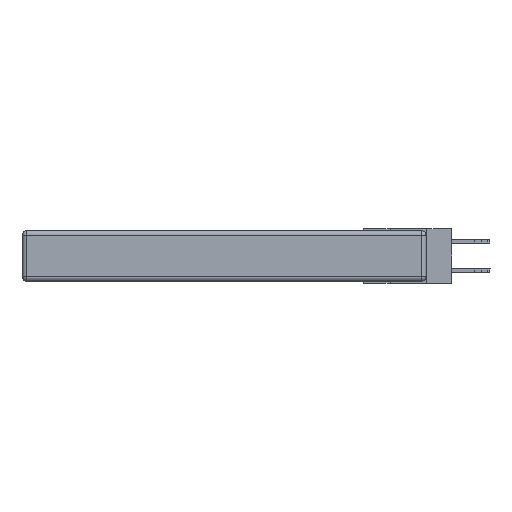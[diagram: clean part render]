
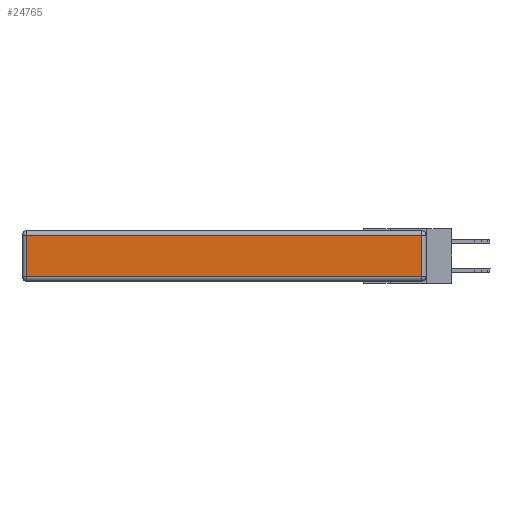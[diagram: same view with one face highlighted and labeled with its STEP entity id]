
A CAD part, left-side view. The second image highlights one B-rep face of the part: STEP entity #24765.
In plain terms, the highlighted planar face has unit normal (-1, 0, 0).
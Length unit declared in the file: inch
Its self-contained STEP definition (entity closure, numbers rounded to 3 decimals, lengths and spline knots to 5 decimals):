
#732 = CARTESIAN_POINT ( 'NONE',  ( 0., 2.75, -0.03 ) ) ;
#1760 = LINE ( 'NONE', #14524, #19308 ) ;
#3325 = VECTOR ( 'NONE', #13319, 39.37008 ) ;
#3763 = FACE_OUTER_BOUND ( 'NONE', #21212, .T. ) ;
#4138 = ORIENTED_EDGE ( 'NONE', *, *, #14907, .T. ) ;
#4961 = VERTEX_POINT ( 'NONE', #27779 ) ;
#6233 = CARTESIAN_POINT ( 'NONE',  ( 0., 2.72, -0.03 ) ) ;
#7363 = CARTESIAN_POINT ( 'NONE',  ( 0., 0., -0.343 ) ) ;
#8431 = VERTEX_POINT ( 'NONE', #20762 ) ;
#9537 = DIRECTION ( 'NONE',  ( 0., 1., 0. ) ) ;
#10157 = LINE ( 'NONE', #19404, #17860 ) ;
#10821 = VERTEX_POINT ( 'NONE', #26288 ) ;
#11032 = CARTESIAN_POINT ( 'NONE',  ( 0., 0.03, -0.343 ) ) ;
#11233 = EDGE_CURVE ( 'NONE', #12426, #10821, #1760, .T. ) ;
#12426 = VERTEX_POINT ( 'NONE', #6233 ) ;
#12771 = LINE ( 'NONE', #11032, #3325 ) ;
#13319 = DIRECTION ( 'NONE',  ( 0., 0., 1. ) ) ;
#14084 = ORIENTED_EDGE ( 'NONE', *, *, #19230, .T. ) ;
#14170 = DIRECTION ( 'NONE',  ( 0., 0., 1. ) ) ;
#14524 = CARTESIAN_POINT ( 'NONE',  ( 0., 2.72, -0.343 ) ) ;
#14707 = DIRECTION ( 'NONE',  ( 0., 0., -1. ) ) ;
#14907 = EDGE_CURVE ( 'NONE', #8431, #12426, #20083, .T. ) ;
#17586 = VECTOR ( 'NONE', #9537, 39.37008 ) ;
#17860 = VECTOR ( 'NONE', #23443, 39.37008 ) ;
#18575 = DIRECTION ( 'NONE',  ( -1., 0., 0. ) ) ;
#18581 = PLANE ( 'NONE',  #25938 ) ;
#19230 = EDGE_CURVE ( 'NONE', #10821, #4961, #10157, .T. ) ;
#19308 = VECTOR ( 'NONE', #14707, 39.37008 ) ;
#19404 = CARTESIAN_POINT ( 'NONE',  ( 0., 0., -0.313 ) ) ;
#20083 = LINE ( 'NONE', #732, #17586 ) ;
#20762 = CARTESIAN_POINT ( 'NONE',  ( 0., 0.03, -0.03 ) ) ;
#21212 = EDGE_LOOP ( 'NONE', ( #14084, #24788, #4138, #22020 ) ) ;
#22020 = ORIENTED_EDGE ( 'NONE', *, *, #11233, .T. ) ;
#22824 = EDGE_CURVE ( 'NONE', #4961, #8431, #12771, .T. ) ;
#23443 = DIRECTION ( 'NONE',  ( 0., -1., 0. ) ) ;
#24765 = ADVANCED_FACE ( 'NONE', ( #3763 ), #18581, .T. ) ;
#24788 = ORIENTED_EDGE ( 'NONE', *, *, #22824, .T. ) ;
#25938 = AXIS2_PLACEMENT_3D ( 'NONE', #7363, #18575, #14170 ) ;
#26288 = CARTESIAN_POINT ( 'NONE',  ( 0., 2.72, -0.313 ) ) ;
#27779 = CARTESIAN_POINT ( 'NONE',  ( 0., 0.03, -0.313 ) ) ;
